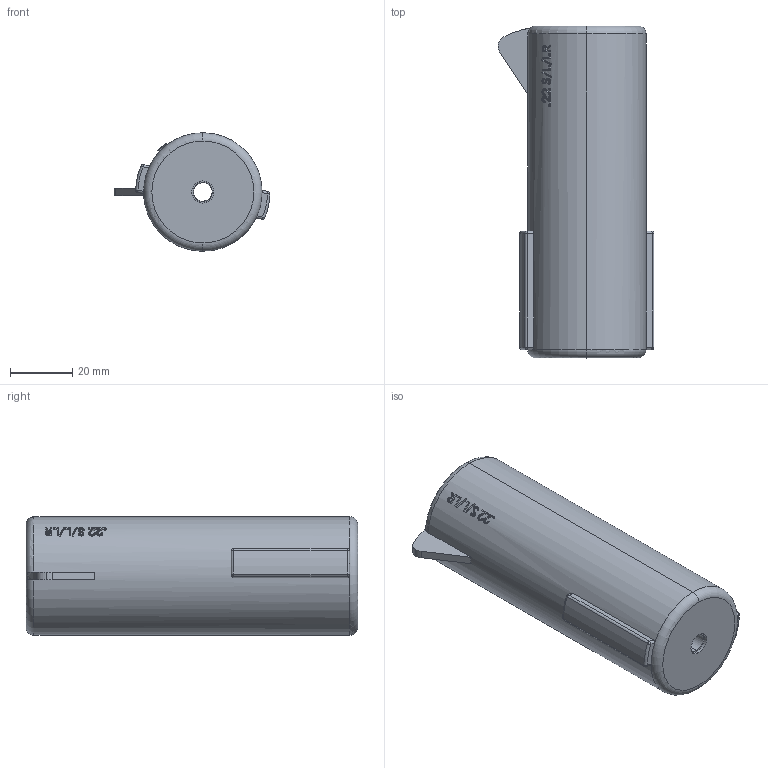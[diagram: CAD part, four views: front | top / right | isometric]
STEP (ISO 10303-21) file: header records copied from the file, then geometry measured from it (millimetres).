
FILE_DESCRIPTION (( 'STEP AP214' ), '1' );
FILE_NAME ('barrel4.STEP', '2013-10-27T06:43:45', ( 'Matt' ), ( '' ), 'SwSTEP 2.0', 'SolidWorks 2013', '' );
FILE_SCHEMA (( 'AUTOMOTIVE_DESIGN' ));
Length unit declared in the file: inch
Products named in the file (1): barrel4
Bounding box: 50.12 x 106.68 x 38.1 mm (x, y, z)
Volume: 119882.7 mm3; surface area: 17853.8 mm2
Topology: 1 solids, 1 shells, 173 faces, 456 edges, 288 vertices
Faces by surface type: bspline 67, plane 52, cylinder 36, torus 8, sphere 8, cone 2
Entity records: 11907 total; most frequent: CARTESIAN_POINT 8290, ORIENTED_EDGE 896, DIRECTION 529, EDGE_CURVE 448, VERTEX_POINT 288, AXIS2_PLACEMENT_3D 210, EDGE_LOOP 186, B_SPLINE_CURVE_WITH_KNOTS 181
